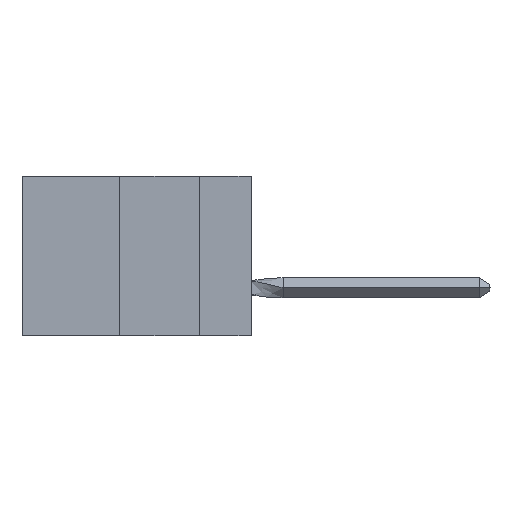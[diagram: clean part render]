
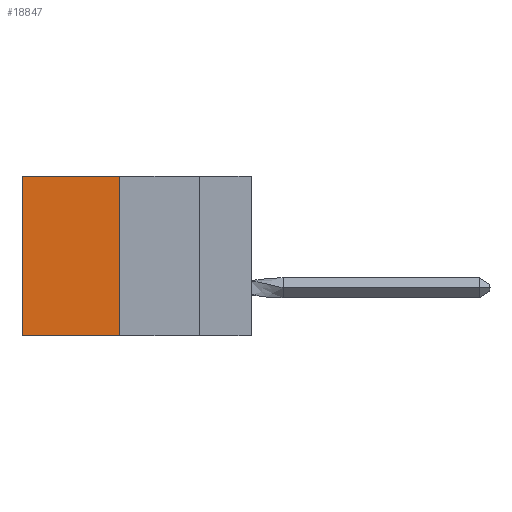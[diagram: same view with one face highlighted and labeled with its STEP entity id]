
A CAD part, left-side view. The second image highlights one B-rep face of the part: STEP entity #18847.
In plain terms, the highlighted planar face has unit normal (-1, 0, 0).
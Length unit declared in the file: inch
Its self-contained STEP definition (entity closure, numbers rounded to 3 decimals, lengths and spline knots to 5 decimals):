
#605 = CARTESIAN_POINT ( 'NONE',  ( 0.305, 0.72, -0.5 ) ) ;
#2640 = VECTOR ( 'NONE', #2725, 39.37008 ) ;
#2725 = DIRECTION ( 'NONE',  ( 0., 0., -1. ) ) ;
#3136 = DIRECTION ( 'NONE',  ( 0., 1., 0. ) ) ;
#3585 = VECTOR ( 'NONE', #8037, 39.37008 ) ;
#4498 = VERTEX_POINT ( 'NONE', #25452 ) ;
#6863 = DIRECTION ( 'NONE',  ( 0., 1., 0. ) ) ;
#6938 = ORIENTED_EDGE ( 'NONE', *, *, #7106, .F. ) ;
#7106 = EDGE_CURVE ( 'NONE', #4498, #17246, #10772, .T. ) ;
#7311 = PLANE ( 'NONE',  #9349 ) ;
#7457 = LINE ( 'NONE', #25344, #16678 ) ;
#7524 = VECTOR ( 'NONE', #3136, 39.37008 ) ;
#7981 = ORIENTED_EDGE ( 'NONE', *, *, #14591, .T. ) ;
#8037 = DIRECTION ( 'NONE',  ( 0., 0., -1. ) ) ;
#9349 = AXIS2_PLACEMENT_3D ( 'NONE', #21856, #11318, #19437 ) ;
#10772 = LINE ( 'NONE', #11300, #7524 ) ;
#11300 = CARTESIAN_POINT ( 'NONE',  ( 0.305, 0.413, -0.5 ) ) ;
#11317 = LINE ( 'NONE', #26363, #3585 ) ;
#11318 = DIRECTION ( 'NONE',  ( 1., 0., 0. ) ) ;
#13194 = CARTESIAN_POINT ( 'NONE',  ( 0.305, 0.72, -0.5 ) ) ;
#13540 = LINE ( 'NONE', #13194, #2640 ) ;
#13918 = EDGE_CURVE ( 'NONE', #25179, #4498, #11317, .T. ) ;
#14567 = FACE_OUTER_BOUND ( 'NONE', #25583, .T. ) ;
#14591 = EDGE_CURVE ( 'NONE', #25179, #23255, #7457, .T. ) ;
#15605 = CARTESIAN_POINT ( 'NONE',  ( 0.305, 0.72, 0. ) ) ;
#16678 = VECTOR ( 'NONE', #6863, 39.37008 ) ;
#17246 = VERTEX_POINT ( 'NONE', #605 ) ;
#18471 = ORIENTED_EDGE ( 'NONE', *, *, #23779, .T. ) ;
#18847 = ADVANCED_FACE ( 'NONE', ( #14567 ), #7311, .F. ) ;
#19437 = DIRECTION ( 'NONE',  ( 0., 0., -1. ) ) ;
#21856 = CARTESIAN_POINT ( 'NONE',  ( 0.305, 0.413, -0.5 ) ) ;
#23255 = VERTEX_POINT ( 'NONE', #15605 ) ;
#23779 = EDGE_CURVE ( 'NONE', #23255, #17246, #13540, .T. ) ;
#24859 = ORIENTED_EDGE ( 'NONE', *, *, #13918, .F. ) ;
#25179 = VERTEX_POINT ( 'NONE', #26094 ) ;
#25344 = CARTESIAN_POINT ( 'NONE',  ( 0.305, 0.413, 0. ) ) ;
#25452 = CARTESIAN_POINT ( 'NONE',  ( 0.305, 0.413, -0.5 ) ) ;
#25583 = EDGE_LOOP ( 'NONE', ( #18471, #6938, #24859, #7981 ) ) ;
#26094 = CARTESIAN_POINT ( 'NONE',  ( 0.305, 0.413, 0. ) ) ;
#26363 = CARTESIAN_POINT ( 'NONE',  ( 0.305, 0.413, -0.5 ) ) ;
